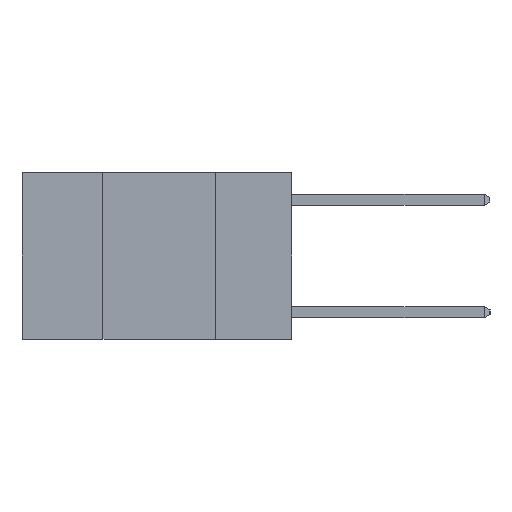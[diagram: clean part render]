
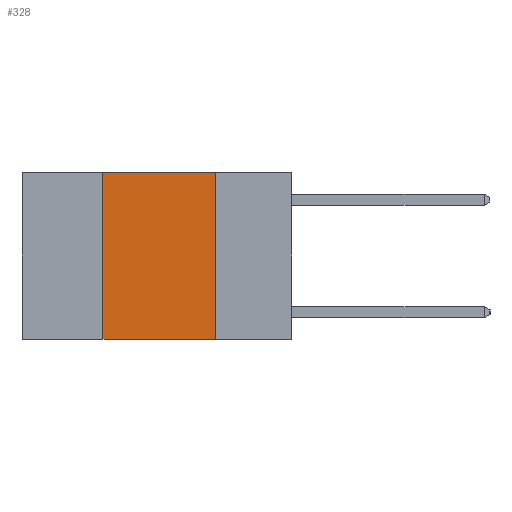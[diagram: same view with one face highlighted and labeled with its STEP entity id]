
A CAD part, left-side view. The second image highlights one B-rep face of the part: STEP entity #328.
In plain terms, the highlighted planar face has unit normal (-1, 0, 0).
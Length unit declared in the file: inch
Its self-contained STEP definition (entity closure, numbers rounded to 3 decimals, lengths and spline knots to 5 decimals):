
#328 = ADVANCED_FACE ( 'NONE', ( #8465 ), #2468, .F. ) ;
#378 = ORIENTED_EDGE ( 'NONE', *, *, #1989, .F. ) ;
#556 = AXIS2_PLACEMENT_3D ( 'NONE', #5439, #3548, #5783 ) ;
#586 = ORIENTED_EDGE ( 'NONE', *, *, #1016, .F. ) ;
#625 = EDGE_CURVE ( 'NONE', #858, #3012, #7523, .T. ) ;
#843 = LINE ( 'NONE', #2837, #4249 ) ;
#858 = VERTEX_POINT ( 'NONE', #7669 ) ;
#1016 = EDGE_CURVE ( 'NONE', #1143, #3012, #3985, .T. ) ;
#1143 = VERTEX_POINT ( 'NONE', #5270 ) ;
#1262 = VERTEX_POINT ( 'NONE', #4118 ) ;
#1989 = EDGE_CURVE ( 'NONE', #1262, #1143, #843, .T. ) ;
#2171 = VECTOR ( 'NONE', #4115, 39.37008 ) ;
#2468 = PLANE ( 'NONE',  #556 ) ;
#2551 = EDGE_CURVE ( 'NONE', #858, #1262, #3085, .T. ) ;
#2801 = CARTESIAN_POINT ( 'NONE',  ( 0., 0.42, 0. ) ) ;
#2837 = CARTESIAN_POINT ( 'NONE',  ( 0., 0.6, 0. ) ) ;
#3012 = VERTEX_POINT ( 'NONE', #7348 ) ;
#3085 = LINE ( 'NONE', #2801, #8199 ) ;
#3296 = DIRECTION ( 'NONE',  ( 0., -1., 0. ) ) ;
#3548 = DIRECTION ( 'NONE',  ( 1., 0., 0. ) ) ;
#3985 = LINE ( 'NONE', #5362, #2171 ) ;
#4115 = DIRECTION ( 'NONE',  ( 0., 0., -1. ) ) ;
#4118 = CARTESIAN_POINT ( 'NONE',  ( 0., 0.42, 0. ) ) ;
#4203 = DIRECTION ( 'NONE',  ( 0., 0., 1. ) ) ;
#4249 = VECTOR ( 'NONE', #3296, 39.37008 ) ;
#5270 = CARTESIAN_POINT ( 'NONE',  ( 0., 0.17, 0. ) ) ;
#5362 = CARTESIAN_POINT ( 'NONE',  ( 0., 0.17, 0. ) ) ;
#5439 = CARTESIAN_POINT ( 'NONE',  ( 0., 0.6, 0. ) ) ;
#5761 = VECTOR ( 'NONE', #8685, 39.37008 ) ;
#5783 = DIRECTION ( 'NONE',  ( 0., 0., -1. ) ) ;
#6708 = CARTESIAN_POINT ( 'NONE',  ( 0., 0.6, -0.37 ) ) ;
#6858 = ORIENTED_EDGE ( 'NONE', *, *, #625, .T. ) ;
#7348 = CARTESIAN_POINT ( 'NONE',  ( 0., 0.17, -0.37 ) ) ;
#7523 = LINE ( 'NONE', #6708, #5761 ) ;
#7669 = CARTESIAN_POINT ( 'NONE',  ( 0., 0.42, -0.37 ) ) ;
#8199 = VECTOR ( 'NONE', #4203, 39.37008 ) ;
#8465 = FACE_OUTER_BOUND ( 'NONE', #8697, .T. ) ;
#8685 = DIRECTION ( 'NONE',  ( 0., -1., 0. ) ) ;
#8697 = EDGE_LOOP ( 'NONE', ( #586, #378, #8717, #6858 ) ) ;
#8717 = ORIENTED_EDGE ( 'NONE', *, *, #2551, .F. ) ;
